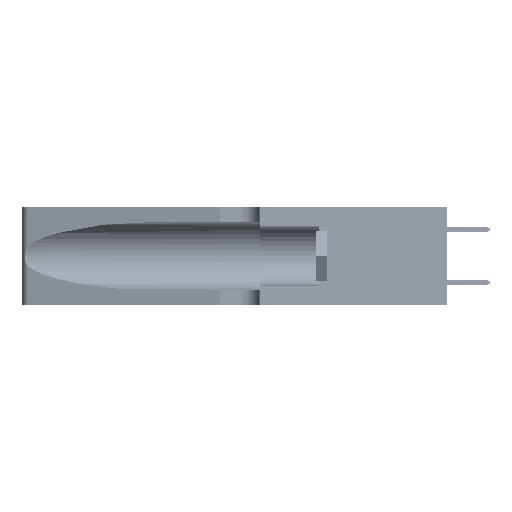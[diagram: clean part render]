
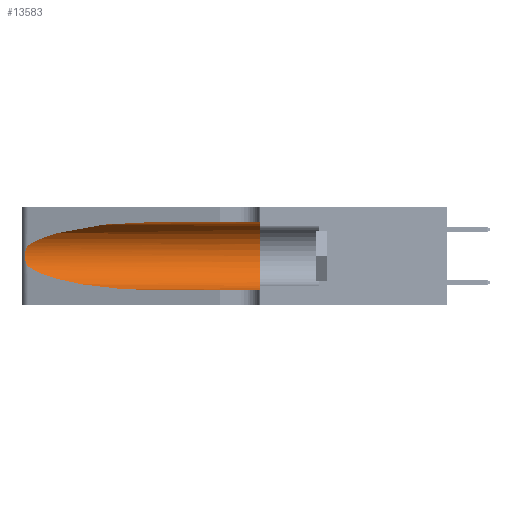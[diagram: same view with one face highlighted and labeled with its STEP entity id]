
A CAD part, left-side view. The second image highlights one B-rep face of the part: STEP entity #13583.
In plain terms, the highlighted cylindrical face has radius 3.308 mm (diameter 6.617 mm), a partial arc.
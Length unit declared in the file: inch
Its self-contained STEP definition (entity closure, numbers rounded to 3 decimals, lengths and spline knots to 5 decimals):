
#202 = CARTESIAN_POINT ( 'NONE',  ( 0.25639, 1.23184, 0.21858 ) ) ;
#921 = B_SPLINE_CURVE_WITH_KNOTS ( 'NONE', 3,
 ( #45663, #4243, #202, #29292, #4415, #33414, #8592, #37598, #12821, #41689, #16998, #45846, #21159, #49986 ),
 .UNSPECIFIED., .F., .F.,
 ( 4, 2, 2, 2, 2, 2, 4 ),
 ( 0., 0.00027, 0.00053, 0.00107, 0.0016, 0.00187, 0.00214 ),
 .UNSPECIFIED. ) ;
#2219 = DIRECTION ( 'NONE',  ( 0., 0., 1. ) ) ;
#2225 = CARTESIAN_POINT ( 'NONE',  ( 0.1305, 0.72297, 0.31525 ) ) ;
#2938 = CARTESIAN_POINT ( 'NONE',  ( 0.2373, 1.15595, 0.08982 ) ) ;
#4243 = CARTESIAN_POINT ( 'NONE',  ( 0.25555, 1.22994, 0.2215 ) ) ;
#4415 = CARTESIAN_POINT ( 'NONE',  ( 0.25854, 1.2359, 0.20912 ) ) ;
#4669 = VERTEX_POINT ( 'NONE', #15501 ) ;
#5268 = EDGE_CURVE ( 'NONE', #38266, #30887, #7417, .T. ) ;
#6161 = FACE_OUTER_BOUND ( 'NONE', #35286, .T. ) ;
#7161 = CARTESIAN_POINT ( 'NONE',  ( 0.1305, 0.72297, 0.05475 ) ) ;
#7277 = VECTOR ( 'NONE', #33014, 39.37008 ) ;
#7417 =( BOUNDED_CURVE ( )  B_SPLINE_CURVE ( 3, ( #15084, #39786, #43937, #19240 ),
 .UNSPECIFIED., .F., .F. ) 
 B_SPLINE_CURVE_WITH_KNOTS ( ( 4, 4 ),
 ( 1.5708, 2.84003 ),
 .UNSPECIFIED. ) 
 CURVE ( )  GEOMETRIC_REPRESENTATION_ITEM ( )  RATIONAL_B_SPLINE_CURVE ( ( 1., 0.87, 0.87, 1. ) ) 
 REPRESENTATION_ITEM ( '' )  );
#8592 = CARTESIAN_POINT ( 'NONE',  ( 0.26075, 1.23896, 0.19203 ) ) ;
#9913 = CARTESIAN_POINT ( 'NONE',  ( 0.25487, 1.22718, 0.22369 ) ) ;
#10523 = EDGE_CURVE ( 'NONE', #39617, #4669, #40167, .T. ) ;
#12821 = CARTESIAN_POINT ( 'NONE',  ( 0.26017, 1.23833, 0.17102 ) ) ;
#13328 = CYLINDRICAL_SURFACE ( 'NONE', #42105, 0.13025 ) ;
#13583 = ADVANCED_FACE ( 'NONE', ( #6161 ), #13328, .F. ) ;
#14392 = AXIS2_PLACEMENT_3D ( 'NONE', #51765, #27148, #2219 ) ;
#15084 = CARTESIAN_POINT ( 'NONE',  ( 0.1305, 0.72297, 0.31525 ) ) ;
#15501 = CARTESIAN_POINT ( 'NONE',  ( 0.1305, 0.35, 0.05475 ) ) ;
#15765 = LINE ( 'NONE', #53472, #7277 ) ;
#16915 = DIRECTION ( 'NONE',  ( 0., 0., -1. ) ) ;
#16998 = CARTESIAN_POINT ( 'NONE',  ( 0.25789, 1.23486, 0.15765 ) ) ;
#19240 = CARTESIAN_POINT ( 'NONE',  ( 0.25487, 1.22718, 0.22369 ) ) ;
#19659 = LINE ( 'NONE', #24546, #20955 ) ;
#20955 = VECTOR ( 'NONE', #53293, 39.37008 ) ;
#21159 = CARTESIAN_POINT ( 'NONE',  ( 0.25555, 1.22993, 0.14849 ) ) ;
#21906 = ORIENTED_EDGE ( 'NONE', *, *, #26393, .T. ) ;
#22168 = ORIENTED_EDGE ( 'NONE', *, *, #50745, .T. ) ;
#24546 = CARTESIAN_POINT ( 'NONE',  ( 0.1305, 1.61858, 0.31525 ) ) ;
#26393 = EDGE_CURVE ( 'NONE', #45155, #4669, #15765, .T. ) ;
#27148 = DIRECTION ( 'NONE',  ( 0., 1., 0. ) ) ;
#29292 = CARTESIAN_POINT ( 'NONE',  ( 0.25787, 1.23484, 0.2124 ) ) ;
#30887 = VERTEX_POINT ( 'NONE', #9913 ) ;
#31121 = ORIENTED_EDGE ( 'NONE', *, *, #33725, .T. ) ;
#31957 = CARTESIAN_POINT ( 'NONE',  ( 0.25487, 1.22718, 0.14631 ) ) ;
#32264 = CARTESIAN_POINT ( 'NONE',  ( 0.1305, 0.35, 0.31525 ) ) ;
#33014 = DIRECTION ( 'NONE',  ( 0., -1., 0. ) ) ;
#33099 = CARTESIAN_POINT ( 'NONE',  ( 0.1305, 0.72297, 0.05475 ) ) ;
#33414 = CARTESIAN_POINT ( 'NONE',  ( 0.26018, 1.23835, 0.19895 ) ) ;
#33725 = EDGE_CURVE ( 'NONE', #52226, #45155, #48016, .T. ) ;
#33731 = ORIENTED_EDGE ( 'NONE', *, *, #10523, .F. ) ;
#34119 = ORIENTED_EDGE ( 'NONE', *, *, #5268, .T. ) ;
#35286 = EDGE_LOOP ( 'NONE', ( #34119, #22168, #31121, #21906, #33731, #46870 ) ) ;
#37598 = CARTESIAN_POINT ( 'NONE',  ( 0.26075, 1.23896, 0.178 ) ) ;
#38266 = VERTEX_POINT ( 'NONE', #2225 ) ;
#39617 = VERTEX_POINT ( 'NONE', #32264 ) ;
#39786 = CARTESIAN_POINT ( 'NONE',  ( 0.18966, 0.96281, 0.31525 ) ) ;
#40167 = CIRCLE ( 'NONE', #14392, 0.13025 ) ;
#41667 = EDGE_CURVE ( 'NONE', #38266, #39617, #19659, .T. ) ;
#41689 = CARTESIAN_POINT ( 'NONE',  ( 0.25856, 1.23593, 0.16098 ) ) ;
#42105 = AXIS2_PLACEMENT_3D ( 'NONE', #45762, #49909, #16915 ) ;
#43937 = CARTESIAN_POINT ( 'NONE',  ( 0.2373, 1.15595, 0.28018 ) ) ;
#45155 = VERTEX_POINT ( 'NONE', #33099 ) ;
#45663 = CARTESIAN_POINT ( 'NONE',  ( 0.25487, 1.22718, 0.22369 ) ) ;
#45762 = CARTESIAN_POINT ( 'NONE',  ( 0.1305, 1.61858, 0.185 ) ) ;
#45846 = CARTESIAN_POINT ( 'NONE',  ( 0.25639, 1.23186, 0.15144 ) ) ;
#46870 = ORIENTED_EDGE ( 'NONE', *, *, #41667, .F. ) ;
#47351 = CARTESIAN_POINT ( 'NONE',  ( 0.25487, 1.22718, 0.14631 ) ) ;
#48016 =( BOUNDED_CURVE ( )  B_SPLINE_CURVE ( 3, ( #31957, #2938, #52450, #7161 ),
 .UNSPECIFIED., .F., .T. ) 
 B_SPLINE_CURVE_WITH_KNOTS ( ( 4, 4 ),
 ( 3.44316, 4.71239 ),
 .UNSPECIFIED. ) 
 CURVE ( )  GEOMETRIC_REPRESENTATION_ITEM ( )  RATIONAL_B_SPLINE_CURVE ( ( 1., 0.87, 0.87, 1. ) ) 
 REPRESENTATION_ITEM ( '' )  );
#49909 = DIRECTION ( 'NONE',  ( 0., -1., 0. ) ) ;
#49986 = CARTESIAN_POINT ( 'NONE',  ( 0.25487, 1.22718, 0.14631 ) ) ;
#50745 = EDGE_CURVE ( 'NONE', #30887, #52226, #921, .T. ) ;
#51765 = CARTESIAN_POINT ( 'NONE',  ( 0.1305, 0.35, 0.185 ) ) ;
#52226 = VERTEX_POINT ( 'NONE', #47351 ) ;
#52450 = CARTESIAN_POINT ( 'NONE',  ( 0.18966, 0.96281, 0.05475 ) ) ;
#53293 = DIRECTION ( 'NONE',  ( 0., -1., 0. ) ) ;
#53472 = CARTESIAN_POINT ( 'NONE',  ( 0.1305, 1.61858, 0.05475 ) ) ;
